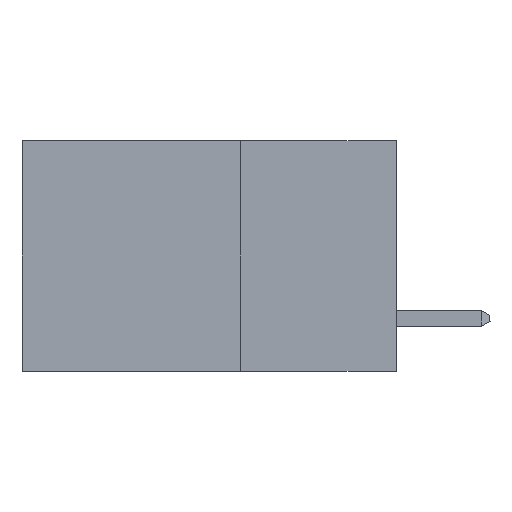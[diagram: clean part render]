
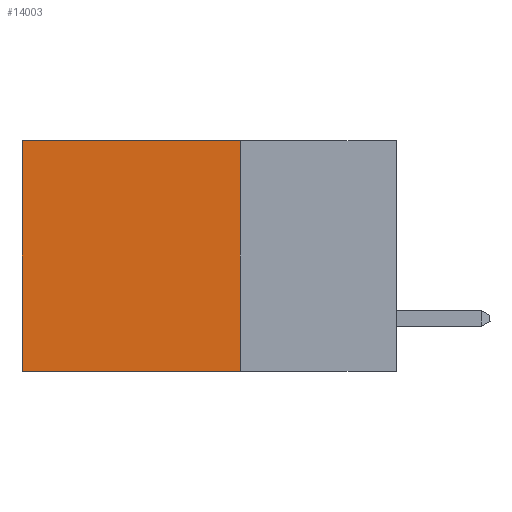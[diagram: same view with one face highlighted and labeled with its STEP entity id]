
A CAD part, left-side view. The second image highlights one B-rep face of the part: STEP entity #14003.
In plain terms, the highlighted planar face has unit normal (-1, 0, 0).
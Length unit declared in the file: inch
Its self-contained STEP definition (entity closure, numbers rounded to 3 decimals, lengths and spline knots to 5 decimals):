
#211 = VERTEX_POINT ( 'NONE', #24974 ) ;
#1928 = ORIENTED_EDGE ( 'NONE', *, *, #19241, .F. ) ;
#2541 = LINE ( 'NONE', #6949, #21291 ) ;
#3010 = PLANE ( 'NONE',  #23462 ) ;
#3951 = VERTEX_POINT ( 'NONE', #6942 ) ;
#4646 = EDGE_CURVE ( 'NONE', #211, #3951, #6781, .T. ) ;
#4887 = DIRECTION ( 'NONE',  ( 0., 0., -1. ) ) ;
#5151 = ORIENTED_EDGE ( 'NONE', *, *, #20627, .F. ) ;
#5331 = ORIENTED_EDGE ( 'NONE', *, *, #28448, .T. ) ;
#6631 = LINE ( 'NONE', #22543, #14133 ) ;
#6781 = LINE ( 'NONE', #20262, #24046 ) ;
#6942 = CARTESIAN_POINT ( 'NONE',  ( 0.298, 0.6, 0. ) ) ;
#6949 = CARTESIAN_POINT ( 'NONE',  ( 0.298, 0.25, -0.37 ) ) ;
#7902 = CARTESIAN_POINT ( 'NONE',  ( 0.298, 0.25, 0. ) ) ;
#8240 = EDGE_LOOP ( 'NONE', ( #5331, #5151, #1928, #10975 ) ) ;
#8286 = VERTEX_POINT ( 'NONE', #12319 ) ;
#9509 = VECTOR ( 'NONE', #4887, 39.37008 ) ;
#10975 = ORIENTED_EDGE ( 'NONE', *, *, #4646, .T. ) ;
#11175 = DIRECTION ( 'NONE',  ( 0., 1., 0. ) ) ;
#12319 = CARTESIAN_POINT ( 'NONE',  ( 0.298, 0.6, -0.37 ) ) ;
#12609 = VERTEX_POINT ( 'NONE', #19799 ) ;
#13916 = FACE_OUTER_BOUND ( 'NONE', #8240, .T. ) ;
#14003 = ADVANCED_FACE ( 'NONE', ( #13916 ), #3010, .F. ) ;
#14133 = VECTOR ( 'NONE', #22649, 39.37008 ) ;
#16239 = CARTESIAN_POINT ( 'NONE',  ( 0.298, 0.6, 0. ) ) ;
#19241 = EDGE_CURVE ( 'NONE', #211, #12609, #6631, .T. ) ;
#19799 = CARTESIAN_POINT ( 'NONE',  ( 0.298, 0.25, -0.37 ) ) ;
#20262 = CARTESIAN_POINT ( 'NONE',  ( 0.298, 0.25, 0. ) ) ;
#20627 = EDGE_CURVE ( 'NONE', #12609, #8286, #2541, .T. ) ;
#21291 = VECTOR ( 'NONE', #25403, 39.37008 ) ;
#21553 = DIRECTION ( 'NONE',  ( 1., 0., 0. ) ) ;
#22543 = CARTESIAN_POINT ( 'NONE',  ( 0.298, 0.25, 0. ) ) ;
#22649 = DIRECTION ( 'NONE',  ( 0., 0., -1. ) ) ;
#23192 = LINE ( 'NONE', #16239, #9509 ) ;
#23462 = AXIS2_PLACEMENT_3D ( 'NONE', #7902, #21553, #23828 ) ;
#23828 = DIRECTION ( 'NONE',  ( 0., 0., -1. ) ) ;
#24046 = VECTOR ( 'NONE', #11175, 39.37008 ) ;
#24974 = CARTESIAN_POINT ( 'NONE',  ( 0.298, 0.25, 0. ) ) ;
#25403 = DIRECTION ( 'NONE',  ( 0., 1., 0. ) ) ;
#28448 = EDGE_CURVE ( 'NONE', #3951, #8286, #23192, .T. ) ;
